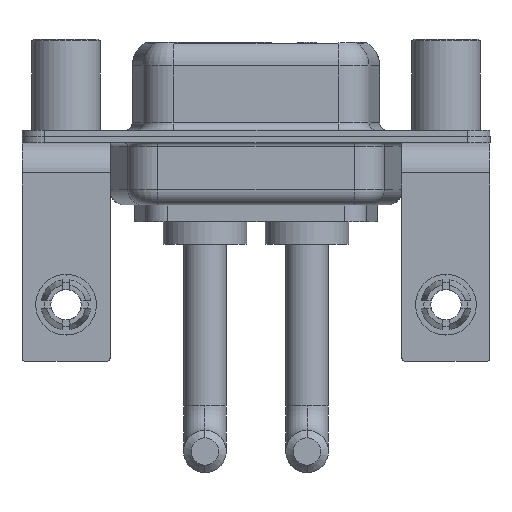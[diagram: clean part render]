
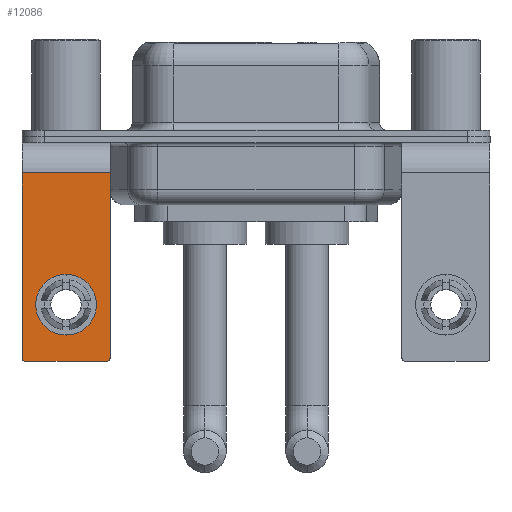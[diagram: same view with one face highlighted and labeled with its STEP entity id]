
A CAD part, front view. The second image highlights one B-rep face of the part: STEP entity #12086.
In plain terms, the highlighted planar face has unit normal (0, -1, 0).
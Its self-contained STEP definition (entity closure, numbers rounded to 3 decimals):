
#187 = EDGE_CURVE ( 'NONE', #13373, #9486, #9467, .T. ) ;
#279 = DIRECTION ( 'NONE',  ( -1., 0., 0. ) ) ;
#590 = DIRECTION ( 'NONE',  ( 0., 0., 1. ) ) ;
#828 = LINE ( 'NONE', #10962, #8434 ) ;
#933 = ORIENTED_EDGE ( 'NONE', *, *, #12775, .T. ) ;
#1260 = VECTOR ( 'NONE', #5081, 1000. ) ;
#1688 = CARTESIAN_POINT ( 'NONE',  ( 2.65, -6.25, -14.8 ) ) ;
#1775 = FACE_BOUND ( 'NONE', #14255, .T. ) ;
#1921 = DIRECTION ( 'NONE',  ( 0., 0., 1. ) ) ;
#2030 = AXIS2_PLACEMENT_3D ( 'NONE', #8939, #15395, #7587 ) ;
#2105 = FACE_OUTER_BOUND ( 'NONE', #10772, .T. ) ;
#2286 = DIRECTION ( 'NONE',  ( 0., 0., 1. ) ) ;
#2464 = CARTESIAN_POINT ( 'NONE',  ( -2.9, -6.25, -14.55 ) ) ;
#2787 = EDGE_CURVE ( 'NONE', #8714, #4577, #4124, .T. ) ;
#2843 = LINE ( 'NONE', #7823, #1260 ) ;
#3188 = DIRECTION ( 'NONE',  ( 0., 1., 0. ) ) ;
#3430 = AXIS2_PLACEMENT_3D ( 'NONE', #11817, #6562, #2286 ) ;
#3476 = AXIS2_PLACEMENT_3D ( 'NONE', #10857, #3188, #8394 ) ;
#3576 = CARTESIAN_POINT ( 'NONE',  ( 0., -6.25, -11.07 ) ) ;
#3684 = CIRCLE ( 'NONE', #5861, 2. ) ;
#3739 = ORIENTED_EDGE ( 'NONE', *, *, #187, .T. ) ;
#4124 = LINE ( 'NONE', #11961, #12449 ) ;
#4577 = VERTEX_POINT ( 'NONE', #13376 ) ;
#4853 = CARTESIAN_POINT ( 'NONE',  ( -2.65, -6.25, -14.8 ) ) ;
#4926 = VERTEX_POINT ( 'NONE', #4853 ) ;
#5081 = DIRECTION ( 'NONE',  ( 0., 0., -1. ) ) ;
#5229 = ORIENTED_EDGE ( 'NONE', *, *, #10592, .F. ) ;
#5457 = AXIS2_PLACEMENT_3D ( 'NONE', #14886, #8569, #1921 ) ;
#5861 = AXIS2_PLACEMENT_3D ( 'NONE', #3576, #8778, #590 ) ;
#6146 = EDGE_CURVE ( 'NONE', #9486, #13373, #3684, .T. ) ;
#6292 = VERTEX_POINT ( 'NONE', #2464 ) ;
#6562 = DIRECTION ( 'NONE',  ( 0., -1., 0. ) ) ;
#6853 = ORIENTED_EDGE ( 'NONE', *, *, #2787, .T. ) ;
#7299 = VERTEX_POINT ( 'NONE', #1688 ) ;
#7587 = DIRECTION ( 'NONE',  ( 0., 0., 1. ) ) ;
#7593 = LINE ( 'NONE', #11478, #10002 ) ;
#7823 = CARTESIAN_POINT ( 'NONE',  ( -2.9, -6.25, -2.4 ) ) ;
#8223 = CARTESIAN_POINT ( 'NONE',  ( 0., -6.25, -13.07 ) ) ;
#8317 = VERTEX_POINT ( 'NONE', #9990 ) ;
#8394 = DIRECTION ( 'NONE',  ( 0., 0., 1. ) ) ;
#8434 = VECTOR ( 'NONE', #14903, 1000. ) ;
#8569 = DIRECTION ( 'NONE',  ( 0., -1., 0. ) ) ;
#8714 = VERTEX_POINT ( 'NONE', #12526 ) ;
#8778 = DIRECTION ( 'NONE',  ( 0., 1., 0. ) ) ;
#8939 = CARTESIAN_POINT ( 'NONE',  ( 2.9, -6.25, -2.4 ) ) ;
#9467 = CIRCLE ( 'NONE', #3476, 2. ) ;
#9486 = VERTEX_POINT ( 'NONE', #10532 ) ;
#9990 = CARTESIAN_POINT ( 'NONE',  ( 2.9, -6.25, -14.55 ) ) ;
#10002 = VECTOR ( 'NONE', #16679, 1000. ) ;
#10532 = CARTESIAN_POINT ( 'NONE',  ( 0., -6.25, -9.07 ) ) ;
#10592 = EDGE_CURVE ( 'NONE', #7299, #4926, #828, .T. ) ;
#10772 = EDGE_LOOP ( 'NONE', ( #15721, #12937, #5229, #933, #14754, #6853 ) ) ;
#10857 = CARTESIAN_POINT ( 'NONE',  ( 0., -6.25, -11.07 ) ) ;
#10962 = CARTESIAN_POINT ( 'NONE',  ( 2.9, -6.25, -14.8 ) ) ;
#11108 = EDGE_CURVE ( 'NONE', #6292, #4926, #15238, .T. ) ;
#11395 = ORIENTED_EDGE ( 'NONE', *, *, #6146, .T. ) ;
#11478 = CARTESIAN_POINT ( 'NONE',  ( 2.9, -6.25, -2.4 ) ) ;
#11817 = CARTESIAN_POINT ( 'NONE',  ( 2.65, -6.25, -14.55 ) ) ;
#11961 = CARTESIAN_POINT ( 'NONE',  ( 2.9, -6.25, -2.4 ) ) ;
#12086 = ADVANCED_FACE ( 'NONE', ( #1775, #2105 ), #14130, .F. ) ;
#12449 = VECTOR ( 'NONE', #279, 1000. ) ;
#12526 = CARTESIAN_POINT ( 'NONE',  ( 2.9, -6.25, -2.4 ) ) ;
#12775 = EDGE_CURVE ( 'NONE', #7299, #8317, #14314, .T. ) ;
#12937 = ORIENTED_EDGE ( 'NONE', *, *, #11108, .T. ) ;
#13192 = EDGE_CURVE ( 'NONE', #4577, #6292, #2843, .T. ) ;
#13373 = VERTEX_POINT ( 'NONE', #8223 ) ;
#13376 = CARTESIAN_POINT ( 'NONE',  ( -2.9, -6.25, -2.4 ) ) ;
#14130 = PLANE ( 'NONE',  #2030 ) ;
#14255 = EDGE_LOOP ( 'NONE', ( #3739, #11395 ) ) ;
#14314 = CIRCLE ( 'NONE', #3430, 0.25 ) ;
#14557 = EDGE_CURVE ( 'NONE', #8714, #8317, #7593, .T. ) ;
#14754 = ORIENTED_EDGE ( 'NONE', *, *, #14557, .F. ) ;
#14886 = CARTESIAN_POINT ( 'NONE',  ( -2.65, -6.25, -14.55 ) ) ;
#14903 = DIRECTION ( 'NONE',  ( -1., 0., 0. ) ) ;
#15238 = CIRCLE ( 'NONE', #5457, 0.25 ) ;
#15395 = DIRECTION ( 'NONE',  ( 0., 1., 0. ) ) ;
#15721 = ORIENTED_EDGE ( 'NONE', *, *, #13192, .T. ) ;
#16679 = DIRECTION ( 'NONE',  ( 0., 0., -1. ) ) ;
